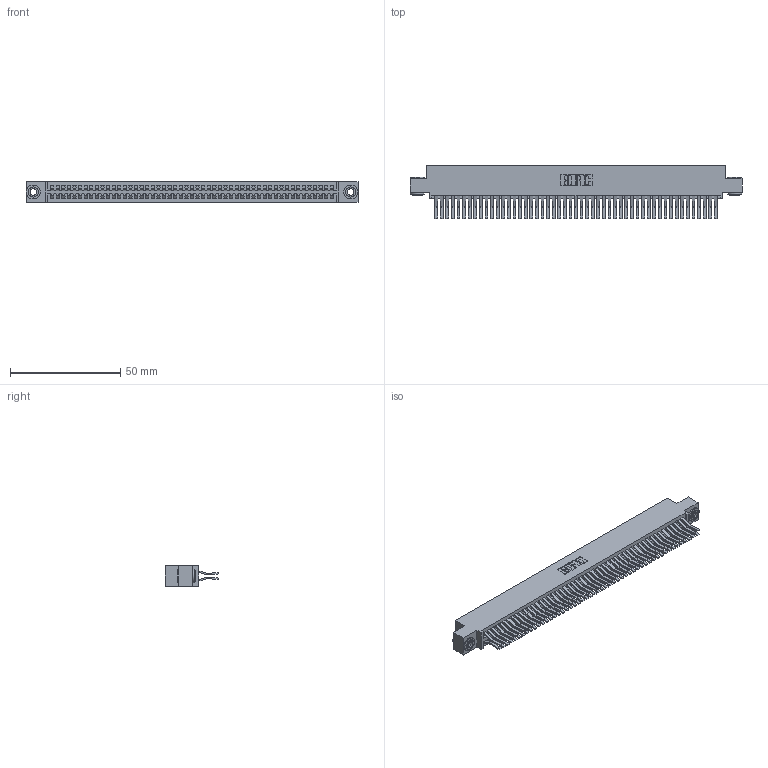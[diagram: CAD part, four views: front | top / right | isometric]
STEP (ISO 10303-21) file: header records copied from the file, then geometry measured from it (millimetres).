
FILE_DESCRIPTION (( 'STEP AP203' ), '1' );
FILE_NAME ('345-102-560-503.STEP', '2018-10-05T21:52:25', ( '' ), ( '' ), 'SwSTEP 2.0', 'SolidWorks 2016', '' );
FILE_SCHEMA (( 'CONFIG_CONTROL_DESIGN' ));
Length unit declared in the file: inch
Products named in the file (4): 345 Part_0.110 Offset - 0.156 Dia-TH; 345-250-002_345-250-002-102; 345-102-560-503; 345-292-001_560 Tail
Assembly tree (105 placements, depth 2):
  345-102-560-503
    345 Part_0.110 Offset - 0.156 Dia-TH
    345-292-001_560 Tail  x102
    345-250-002_345-250-002-102  x2
Bounding box: 150.75 x 24.45 x 9.4 mm (x, y, z)
Volume: 15342.1 mm3; surface area: 24869.7 mm2
Topology: 105 solids, 105 shells, 5472 faces, 16239 edges, 10686 vertices
Faces by surface type: plane 3460, cylinder 2004, cone 8
Entity records: 39674 total; most frequent: CARTESIAN_POINT 6619, ORIENTED_EDGE 6546, DIRECTION 5859, EDGE_CURVE 3273, LINE 2909, VECTOR 2909, VERTEX_POINT 2178, AXIS2_PLACEMENT_3D 1475
